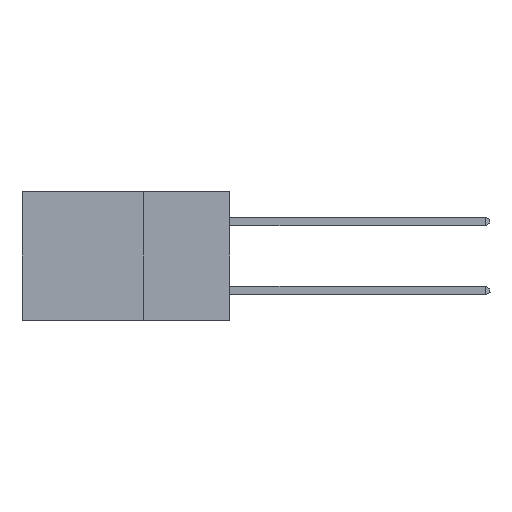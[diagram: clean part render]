
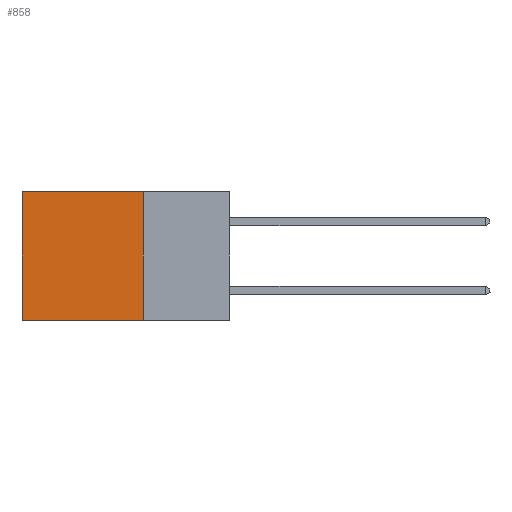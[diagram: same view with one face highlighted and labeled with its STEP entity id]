
A CAD part, left-side view. The second image highlights one B-rep face of the part: STEP entity #858.
In plain terms, the highlighted planar face has unit normal (-1, 0, 0).
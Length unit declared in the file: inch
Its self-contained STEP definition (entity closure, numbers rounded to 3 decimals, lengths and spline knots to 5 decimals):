
#285 = EDGE_CURVE ( 'NONE', #20898, #5690, #5399, .T. ) ;
#627 = VERTEX_POINT ( 'NONE', #12166 ) ;
#858 = ADVANCED_FACE ( 'NONE', ( #19569 ), #9777, .F. ) ;
#1162 = CARTESIAN_POINT ( 'NONE',  ( 0.298, 0.25, 0. ) ) ;
#1503 = VERTEX_POINT ( 'NONE', #6571 ) ;
#3348 = ORIENTED_EDGE ( 'NONE', *, *, #22876, .T. ) ;
#5399 = LINE ( 'NONE', #1162, #16052 ) ;
#5690 = VERTEX_POINT ( 'NONE', #8689 ) ;
#6571 = CARTESIAN_POINT ( 'NONE',  ( 0.298, 0.6, -0.37 ) ) ;
#7417 = AXIS2_PLACEMENT_3D ( 'NONE', #22685, #9469, #13173 ) ;
#7536 = DIRECTION ( 'NONE',  ( 0., 1., 0. ) ) ;
#8580 = ORIENTED_EDGE ( 'NONE', *, *, #22419, .F. ) ;
#8689 = CARTESIAN_POINT ( 'NONE',  ( 0.298, 0.25, -0.37 ) ) ;
#9469 = DIRECTION ( 'NONE',  ( 1., 0., 0. ) ) ;
#9666 = CARTESIAN_POINT ( 'NONE',  ( 0.298, 0.25, 0. ) ) ;
#9777 = PLANE ( 'NONE',  #7417 ) ;
#10989 = CARTESIAN_POINT ( 'NONE',  ( 0.298, 0.25, 0. ) ) ;
#11508 = VECTOR ( 'NONE', #22493, 39.37008 ) ;
#11709 = LINE ( 'NONE', #18673, #13970 ) ;
#12166 = CARTESIAN_POINT ( 'NONE',  ( 0.298, 0.6, 0. ) ) ;
#12610 = DIRECTION ( 'NONE',  ( 0., 0., -1. ) ) ;
#12657 = LINE ( 'NONE', #9666, #11508 ) ;
#13173 = DIRECTION ( 'NONE',  ( 0., 0., -1. ) ) ;
#13970 = VECTOR ( 'NONE', #7536, 39.37008 ) ;
#16052 = VECTOR ( 'NONE', #21575, 39.37008 ) ;
#16395 = ORIENTED_EDGE ( 'NONE', *, *, #285, .F. ) ;
#17400 = VECTOR ( 'NONE', #12610, 39.37008 ) ;
#18673 = CARTESIAN_POINT ( 'NONE',  ( 0.298, 0.25, -0.37 ) ) ;
#19569 = FACE_OUTER_BOUND ( 'NONE', #21501, .T. ) ;
#20361 = LINE ( 'NONE', #23542, #17400 ) ;
#20898 = VERTEX_POINT ( 'NONE', #10989 ) ;
#21501 = EDGE_LOOP ( 'NONE', ( #3348, #8580, #16395, #22209 ) ) ;
#21575 = DIRECTION ( 'NONE',  ( 0., 0., -1. ) ) ;
#21767 = EDGE_CURVE ( 'NONE', #20898, #627, #12657, .T. ) ;
#22209 = ORIENTED_EDGE ( 'NONE', *, *, #21767, .T. ) ;
#22419 = EDGE_CURVE ( 'NONE', #5690, #1503, #11709, .T. ) ;
#22493 = DIRECTION ( 'NONE',  ( 0., 1., 0. ) ) ;
#22685 = CARTESIAN_POINT ( 'NONE',  ( 0.298, 0.25, 0. ) ) ;
#22876 = EDGE_CURVE ( 'NONE', #627, #1503, #20361, .T. ) ;
#23542 = CARTESIAN_POINT ( 'NONE',  ( 0.298, 0.6, 0. ) ) ;
